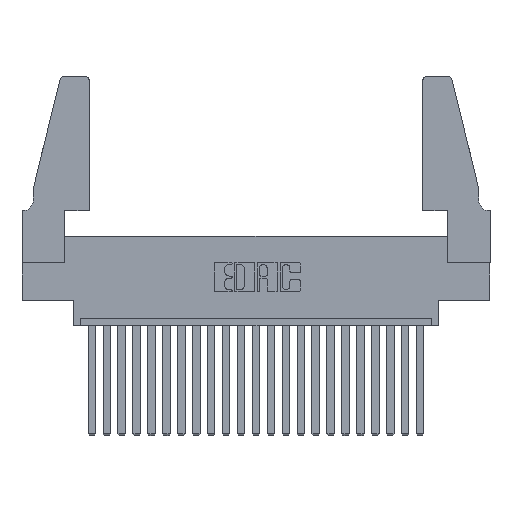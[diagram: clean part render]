
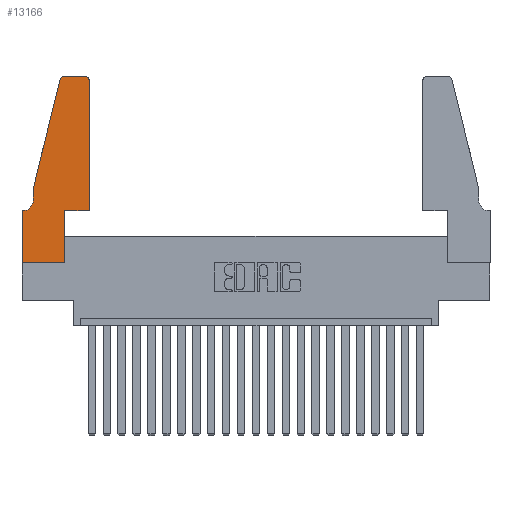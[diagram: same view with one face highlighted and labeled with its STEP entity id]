
A CAD part, top view. The second image highlights one B-rep face of the part: STEP entity #13166.
In plain terms, the highlighted planar face has unit normal (0, 0, 1).
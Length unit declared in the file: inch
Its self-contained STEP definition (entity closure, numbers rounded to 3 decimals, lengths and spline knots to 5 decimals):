
#38 = VERTEX_POINT ( 'NONE', #7616 ) ;
#193 = DIRECTION ( 'NONE',  ( 1., 0., 0. ) ) ;
#502 = CARTESIAN_POINT ( 'NONE',  ( 0.0755, 0.35, 0.37 ) ) ;
#534 = LINE ( 'NONE', #8640, #18068 ) ;
#1070 = ORIENTED_EDGE ( 'NONE', *, *, #15311, .T. ) ;
#1216 = EDGE_CURVE ( 'NONE', #38, #21600, #10386, .T. ) ;
#1796 = LINE ( 'NONE', #4201, #11064 ) ;
#1908 = EDGE_LOOP ( 'NONE', ( #8911, #1070, #14829, #11893, #20737, #19180, #19375, #16102, #5698, #3625, #8217, #19132 ) ) ;
#2267 = DIRECTION ( 'NONE',  ( 0., 1., 0. ) ) ;
#2300 = CIRCLE ( 'NONE', #17502, 0.07 ) ;
#2408 = DIRECTION ( 'NONE',  ( 0., 0., 1. ) ) ;
#2423 = VERTEX_POINT ( 'NONE', #14230 ) ;
#2873 = DIRECTION ( 'NONE',  ( 0., 0., -1. ) ) ;
#3154 = VECTOR ( 'NONE', #6036, 39.37008 ) ;
#3625 = ORIENTED_EDGE ( 'NONE', *, *, #16046, .T. ) ;
#3680 = VERTEX_POINT ( 'NONE', #20810 ) ;
#3708 = VERTEX_POINT ( 'NONE', #3814 ) ;
#3725 = CARTESIAN_POINT ( 'NONE',  ( 0.0755, 0.42, 0.37 ) ) ;
#3783 = CARTESIAN_POINT ( 'NONE',  ( 0.4505, 0.35, 0.37 ) ) ;
#3814 = CARTESIAN_POINT ( 'NONE',  ( 0., 0., 0.37 ) ) ;
#4063 = LINE ( 'NONE', #14726, #8056 ) ;
#4201 = CARTESIAN_POINT ( 'NONE',  ( 0.2865, 0.35, 0.37 ) ) ;
#4444 = CARTESIAN_POINT ( 'NONE',  ( 0.0055, 0.42, 0.37 ) ) ;
#4449 = CARTESIAN_POINT ( 'NONE',  ( 0.0755, 0.5, 0.37 ) ) ;
#4598 = CARTESIAN_POINT ( 'NONE',  ( 0.0755, 0.5, 0.37 ) ) ;
#4608 = DIRECTION ( 'NONE',  ( -1., 0., 0. ) ) ;
#4972 = EDGE_CURVE ( 'NONE', #13952, #5927, #15427, .T. ) ;
#5698 = ORIENTED_EDGE ( 'NONE', *, *, #7420, .T. ) ;
#5927 = VERTEX_POINT ( 'NONE', #17475 ) ;
#6036 = DIRECTION ( 'NONE',  ( 1., 0., 0. ) ) ;
#6488 = AXIS2_PLACEMENT_3D ( 'NONE', #20268, #20338, #8534 ) ;
#6592 = LINE ( 'NONE', #17621, #11846 ) ;
#7028 = DIRECTION ( 'NONE',  ( 0., 1., 0. ) ) ;
#7073 = EDGE_CURVE ( 'NONE', #21600, #3708, #6592, .T. ) ;
#7081 = LINE ( 'NONE', #3783, #10019 ) ;
#7420 = EDGE_CURVE ( 'NONE', #3680, #14210, #1796, .T. ) ;
#7437 = CIRCLE ( 'NONE', #20568, 0.03 ) ;
#7589 = EDGE_CURVE ( 'NONE', #11377, #7923, #14032, .T. ) ;
#7616 = CARTESIAN_POINT ( 'NONE',  ( 0.0055, 0.35, 0.37 ) ) ;
#7793 = CARTESIAN_POINT ( 'NONE',  ( 0.4505, 1.22, 0.37 ) ) ;
#7872 = CARTESIAN_POINT ( 'NONE',  ( 0.284, 1.25, 0.37 ) ) ;
#7923 = VERTEX_POINT ( 'NONE', #4598 ) ;
#8056 = VECTOR ( 'NONE', #4608, 39.37008 ) ;
#8217 = ORIENTED_EDGE ( 'NONE', *, *, #11054, .T. ) ;
#8534 = DIRECTION ( 'NONE',  ( 1., 0., 0. ) ) ;
#8640 = CARTESIAN_POINT ( 'NONE',  ( 0., 0., 0.37 ) ) ;
#8911 = ORIENTED_EDGE ( 'NONE', *, *, #13505, .T. ) ;
#9595 = VECTOR ( 'NONE', #21663, 39.37008 ) ;
#10019 = VECTOR ( 'NONE', #7028, 39.37008 ) ;
#10080 = CARTESIAN_POINT ( 'NONE',  ( 0.0755, 0.5, 0.37 ) ) ;
#10302 = PLANE ( 'NONE',  #6488 ) ;
#10386 = LINE ( 'NONE', #502, #20488 ) ;
#11054 = EDGE_CURVE ( 'NONE', #2423, #13952, #7081, .T. ) ;
#11064 = VECTOR ( 'NONE', #2267, 39.37008 ) ;
#11237 = DIRECTION ( 'NONE',  ( 0., -1., 0. ) ) ;
#11377 = VERTEX_POINT ( 'NONE', #17461 ) ;
#11386 = CARTESIAN_POINT ( 'NONE',  ( 0.2865, 0.35, 0.37 ) ) ;
#11846 = VECTOR ( 'NONE', #11237, 39.37008 ) ;
#11893 = ORIENTED_EDGE ( 'NONE', *, *, #18445, .T. ) ;
#12374 = DIRECTION ( 'NONE',  ( 1., 0., 0. ) ) ;
#12536 = CARTESIAN_POINT ( 'NONE',  ( 0.284, 1.22, 0.37 ) ) ;
#12906 = CARTESIAN_POINT ( 'NONE',  ( 0.4505, 0.35, 0.37 ) ) ;
#13073 = DIRECTION ( 'NONE',  ( -1., 0., 0. ) ) ;
#13166 = ADVANCED_FACE ( 'NONE', ( #14390 ), #10302, .T. ) ;
#13505 = EDGE_CURVE ( 'NONE', #5927, #21281, #4063, .T. ) ;
#13952 = VERTEX_POINT ( 'NONE', #7793 ) ;
#14032 = LINE ( 'NONE', #4449, #9595 ) ;
#14173 = CARTESIAN_POINT ( 'NONE',  ( 0.4205, 1.22, 0.37 ) ) ;
#14210 = VERTEX_POINT ( 'NONE', #11386 ) ;
#14230 = CARTESIAN_POINT ( 'NONE',  ( 0.4505, 0.35, 0.37 ) ) ;
#14390 = FACE_OUTER_BOUND ( 'NONE', #1908, .T. ) ;
#14441 = AXIS2_PLACEMENT_3D ( 'NONE', #14173, #20989, #17467 ) ;
#14513 = DIRECTION ( 'NONE',  ( 0., -1., 0. ) ) ;
#14726 = CARTESIAN_POINT ( 'NONE',  ( 0.2605, 1.25, 0.37 ) ) ;
#14829 = ORIENTED_EDGE ( 'NONE', *, *, #7589, .T. ) ;
#15226 = EDGE_CURVE ( 'NONE', #3708, #3680, #534, .T. ) ;
#15311 = EDGE_CURVE ( 'NONE', #21281, #11377, #7437, .T. ) ;
#15427 = CIRCLE ( 'NONE', #14441, 0.03 ) ;
#15489 = LINE ( 'NONE', #10080, #19254 ) ;
#15706 = VERTEX_POINT ( 'NONE', #3725 ) ;
#16046 = EDGE_CURVE ( 'NONE', #14210, #2423, #19878, .T. ) ;
#16102 = ORIENTED_EDGE ( 'NONE', *, *, #15226, .T. ) ;
#16719 = EDGE_CURVE ( 'NONE', #15706, #38, #2300, .T. ) ;
#17461 = CARTESIAN_POINT ( 'NONE',  ( 0.25487, 1.22718, 0.37 ) ) ;
#17467 = DIRECTION ( 'NONE',  ( 1., 0., 0. ) ) ;
#17475 = CARTESIAN_POINT ( 'NONE',  ( 0.4205, 1.25, 0.37 ) ) ;
#17502 = AXIS2_PLACEMENT_3D ( 'NONE', #4444, #2873, #13073 ) ;
#17621 = CARTESIAN_POINT ( 'NONE',  ( 0., 0., 0.37 ) ) ;
#18068 = VECTOR ( 'NONE', #193, 39.37008 ) ;
#18445 = EDGE_CURVE ( 'NONE', #7923, #15706, #15489, .T. ) ;
#19114 = DIRECTION ( 'NONE',  ( -1., 0., 0. ) ) ;
#19132 = ORIENTED_EDGE ( 'NONE', *, *, #4972, .T. ) ;
#19180 = ORIENTED_EDGE ( 'NONE', *, *, #1216, .T. ) ;
#19254 = VECTOR ( 'NONE', #14513, 39.37008 ) ;
#19375 = ORIENTED_EDGE ( 'NONE', *, *, #7073, .T. ) ;
#19878 = LINE ( 'NONE', #12906, #3154 ) ;
#20268 = CARTESIAN_POINT ( 'NONE',  ( 0., 0.35, 0.37 ) ) ;
#20338 = DIRECTION ( 'NONE',  ( 0., 0., 1. ) ) ;
#20488 = VECTOR ( 'NONE', #19114, 39.37008 ) ;
#20568 = AXIS2_PLACEMENT_3D ( 'NONE', #12536, #2408, #12374 ) ;
#20737 = ORIENTED_EDGE ( 'NONE', *, *, #16719, .T. ) ;
#20810 = CARTESIAN_POINT ( 'NONE',  ( 0.2865, 0., 0.37 ) ) ;
#20989 = DIRECTION ( 'NONE',  ( 0., 0., 1. ) ) ;
#21082 = CARTESIAN_POINT ( 'NONE',  ( 0., 0.35, 0.37 ) ) ;
#21281 = VERTEX_POINT ( 'NONE', #7872 ) ;
#21600 = VERTEX_POINT ( 'NONE', #21082 ) ;
#21663 = DIRECTION ( 'NONE',  ( -0.239, -0.971, 0. ) ) ;
